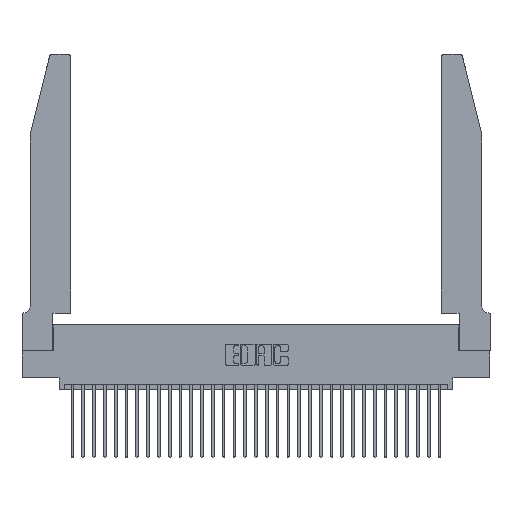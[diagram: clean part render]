
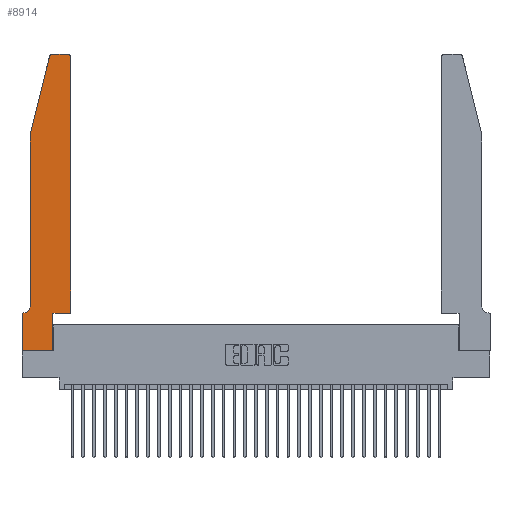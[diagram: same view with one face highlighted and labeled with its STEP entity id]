
A CAD part, top view. The second image highlights one B-rep face of the part: STEP entity #8914.
In plain terms, the highlighted planar face has unit normal (0, 0, 1).
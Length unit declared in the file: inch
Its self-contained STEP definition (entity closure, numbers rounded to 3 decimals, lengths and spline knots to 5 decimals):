
#1072 = ORIENTED_EDGE ( 'NONE', *, *, #21112, .T. ) ;
#1686 = CARTESIAN_POINT ( 'NONE',  ( 0.0055, 0.42, 0.37 ) ) ;
#2506 = LINE ( 'NONE', #6814, #15614 ) ;
#2544 = VECTOR ( 'NONE', #23355, 39.37008 ) ;
#3416 = VERTEX_POINT ( 'NONE', #14731 ) ;
#4288 = LINE ( 'NONE', #5128, #30799 ) ;
#4324 = DIRECTION ( 'NONE',  ( -1., 0., 0. ) ) ;
#4326 = VERTEX_POINT ( 'NONE', #23210 ) ;
#4724 = ORIENTED_EDGE ( 'NONE', *, *, #7189, .T. ) ;
#4789 = LINE ( 'NONE', #18386, #10197 ) ;
#5128 = CARTESIAN_POINT ( 'NONE',  ( 0.2865, 0.35, 0.37 ) ) ;
#5273 = CARTESIAN_POINT ( 'NONE',  ( 0.4505, 2.72, 0.37 ) ) ;
#5300 = CARTESIAN_POINT ( 'NONE',  ( 0.2605, 2.75, 0.37 ) ) ;
#5311 = FACE_OUTER_BOUND ( 'NONE', #30284, .T. ) ;
#5515 = AXIS2_PLACEMENT_3D ( 'NONE', #1686, #19875, #4324 ) ;
#5852 = LINE ( 'NONE', #6725, #33059 ) ;
#6175 = CARTESIAN_POINT ( 'NONE',  ( 0.0755, 2., 0.37 ) ) ;
#6239 = VERTEX_POINT ( 'NONE', #13109 ) ;
#6265 = EDGE_CURVE ( 'NONE', #20481, #6239, #25961, .T. ) ;
#6291 = PLANE ( 'NONE',  #13426 ) ;
#6582 = CARTESIAN_POINT ( 'NONE',  ( 0.2865, 0.35, 0.37 ) ) ;
#6725 = CARTESIAN_POINT ( 'NONE',  ( 0.4505, 0.35, 0.37 ) ) ;
#6814 = CARTESIAN_POINT ( 'NONE',  ( 0., 0., 0.37 ) ) ;
#7189 = EDGE_CURVE ( 'NONE', #12287, #4326, #5852, .T. ) ;
#7785 = VERTEX_POINT ( 'NONE', #11901 ) ;
#7845 = EDGE_CURVE ( 'NONE', #31691, #20481, #2506, .T. ) ;
#8130 = DIRECTION ( 'NONE',  ( -1., 0., 0. ) ) ;
#8914 = ADVANCED_FACE ( 'NONE', ( #5311 ), #6291, .T. ) ;
#8925 = ORIENTED_EDGE ( 'NONE', *, *, #27516, .T. ) ;
#9115 = VECTOR ( 'NONE', #16932, 39.37008 ) ;
#9503 = CARTESIAN_POINT ( 'NONE',  ( 0.4505, 0.35, 0.37 ) ) ;
#9744 = CARTESIAN_POINT ( 'NONE',  ( 0.284, 2.72, 0.37 ) ) ;
#10197 = VECTOR ( 'NONE', #8130, 39.37008 ) ;
#10475 = EDGE_CURVE ( 'NONE', #17887, #12743, #30104, .T. ) ;
#11423 = ORIENTED_EDGE ( 'NONE', *, *, #32188, .T. ) ;
#11591 = CARTESIAN_POINT ( 'NONE',  ( 0., 0.35, 0.37 ) ) ;
#11852 = DIRECTION ( 'NONE',  ( 0., 0., 1. ) ) ;
#11901 = CARTESIAN_POINT ( 'NONE',  ( 0.284, 2.75, 0.37 ) ) ;
#12287 = VERTEX_POINT ( 'NONE', #6582 ) ;
#12376 = DIRECTION ( 'NONE',  ( 1., 0., 0. ) ) ;
#12743 = VERTEX_POINT ( 'NONE', #13656 ) ;
#13109 = CARTESIAN_POINT ( 'NONE',  ( 0.2865, 0., 0.37 ) ) ;
#13303 = VERTEX_POINT ( 'NONE', #6175 ) ;
#13426 = AXIS2_PLACEMENT_3D ( 'NONE', #11591, #29358, #14198 ) ;
#13490 = EDGE_CURVE ( 'NONE', #3416, #13303, #15678, .T. ) ;
#13656 = CARTESIAN_POINT ( 'NONE',  ( 0.0055, 0.35, 0.37 ) ) ;
#14198 = DIRECTION ( 'NONE',  ( 1., 0., 0. ) ) ;
#14731 = CARTESIAN_POINT ( 'NONE',  ( 0.25487, 2.72718, 0.37 ) ) ;
#14733 = ORIENTED_EDGE ( 'NONE', *, *, #22229, .T. ) ;
#14950 = DIRECTION ( 'NONE',  ( -0.239, -0.971, 0. ) ) ;
#15077 = ORIENTED_EDGE ( 'NONE', *, *, #10475, .T. ) ;
#15614 = VECTOR ( 'NONE', #27297, 39.37008 ) ;
#15678 = LINE ( 'NONE', #27540, #28343 ) ;
#15854 = VERTEX_POINT ( 'NONE', #5273 ) ;
#16429 = ORIENTED_EDGE ( 'NONE', *, *, #31108, .T. ) ;
#16932 = DIRECTION ( 'NONE',  ( 0., -1., 0. ) ) ;
#17887 = VERTEX_POINT ( 'NONE', #23085 ) ;
#18213 = ORIENTED_EDGE ( 'NONE', *, *, #13490, .T. ) ;
#18331 = CARTESIAN_POINT ( 'NONE',  ( 0., 0., 0.37 ) ) ;
#18386 = CARTESIAN_POINT ( 'NONE',  ( 0.0755, 0.35, 0.37 ) ) ;
#18569 = ORIENTED_EDGE ( 'NONE', *, *, #22880, .T. ) ;
#19254 = VECTOR ( 'NONE', #23431, 39.37008 ) ;
#19590 = AXIS2_PLACEMENT_3D ( 'NONE', #9744, #27527, #12376 ) ;
#19875 = DIRECTION ( 'NONE',  ( 0., 0., -1. ) ) ;
#19882 = CARTESIAN_POINT ( 'NONE',  ( 0., 0.35, 0.37 ) ) ;
#19950 = LINE ( 'NONE', #24490, #9115 ) ;
#20481 = VERTEX_POINT ( 'NONE', #20983 ) ;
#20619 = LINE ( 'NONE', #9503, #26553 ) ;
#20983 = CARTESIAN_POINT ( 'NONE',  ( 0., 0., 0.37 ) ) ;
#21112 = EDGE_CURVE ( 'NONE', #12743, #31691, #4789, .T. ) ;
#21197 = CARTESIAN_POINT ( 'NONE',  ( 0.4205, 2.75, 0.37 ) ) ;
#21621 = LINE ( 'NONE', #5300, #2544 ) ;
#22229 = EDGE_CURVE ( 'NONE', #6239, #12287, #4288, .T. ) ;
#22880 = EDGE_CURVE ( 'NONE', #15854, #31965, #32725, .T. ) ;
#23085 = CARTESIAN_POINT ( 'NONE',  ( 0.0755, 0.42, 0.37 ) ) ;
#23195 = DIRECTION ( 'NONE',  ( 0., 1., 0. ) ) ;
#23210 = CARTESIAN_POINT ( 'NONE',  ( 0.4505, 0.35, 0.37 ) ) ;
#23355 = DIRECTION ( 'NONE',  ( -1., 0., 0. ) ) ;
#23431 = DIRECTION ( 'NONE',  ( 1., 0., 0. ) ) ;
#23872 = ORIENTED_EDGE ( 'NONE', *, *, #7845, .T. ) ;
#24314 = AXIS2_PLACEMENT_3D ( 'NONE', #27035, #11852, #29590 ) ;
#24358 = ORIENTED_EDGE ( 'NONE', *, *, #30881, .T. ) ;
#24490 = CARTESIAN_POINT ( 'NONE',  ( 0.0755, 2., 0.37 ) ) ;
#24684 = DIRECTION ( 'NONE',  ( 1., 0., 0. ) ) ;
#25961 = LINE ( 'NONE', #18331, #19254 ) ;
#26553 = VECTOR ( 'NONE', #29869, 39.37008 ) ;
#27035 = CARTESIAN_POINT ( 'NONE',  ( 0.4205, 2.72, 0.37 ) ) ;
#27297 = DIRECTION ( 'NONE',  ( 0., -1., 0. ) ) ;
#27423 = ORIENTED_EDGE ( 'NONE', *, *, #6265, .T. ) ;
#27516 = EDGE_CURVE ( 'NONE', #4326, #15854, #20619, .T. ) ;
#27527 = DIRECTION ( 'NONE',  ( 0., 0., 1. ) ) ;
#27540 = CARTESIAN_POINT ( 'NONE',  ( 0.0755, 2., 0.37 ) ) ;
#27926 = CIRCLE ( 'NONE', #19590, 0.03 ) ;
#28343 = VECTOR ( 'NONE', #14950, 39.37008 ) ;
#29358 = DIRECTION ( 'NONE',  ( 0., 0., 1. ) ) ;
#29590 = DIRECTION ( 'NONE',  ( 1., 0., 0. ) ) ;
#29869 = DIRECTION ( 'NONE',  ( 0., 1., 0. ) ) ;
#30104 = CIRCLE ( 'NONE', #5515, 0.07 ) ;
#30284 = EDGE_LOOP ( 'NONE', ( #16429, #24358, #18213, #11423, #15077, #1072, #23872, #27423, #14733, #4724, #8925, #18569 ) ) ;
#30799 = VECTOR ( 'NONE', #23195, 39.37008 ) ;
#30881 = EDGE_CURVE ( 'NONE', #7785, #3416, #27926, .T. ) ;
#31108 = EDGE_CURVE ( 'NONE', #31965, #7785, #21621, .T. ) ;
#31691 = VERTEX_POINT ( 'NONE', #19882 ) ;
#31965 = VERTEX_POINT ( 'NONE', #21197 ) ;
#32188 = EDGE_CURVE ( 'NONE', #13303, #17887, #19950, .T. ) ;
#32725 = CIRCLE ( 'NONE', #24314, 0.03 ) ;
#33059 = VECTOR ( 'NONE', #24684, 39.37008 ) ;
